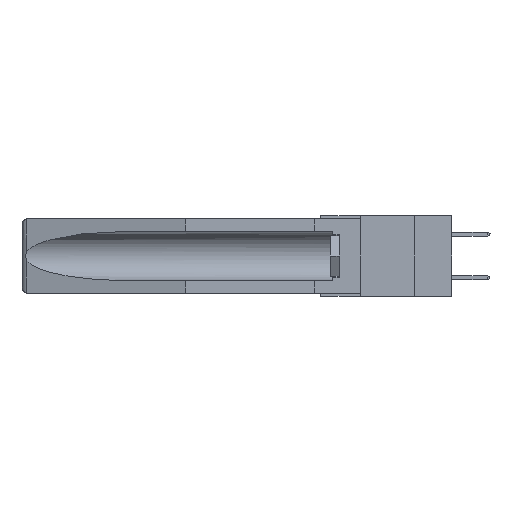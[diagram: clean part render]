
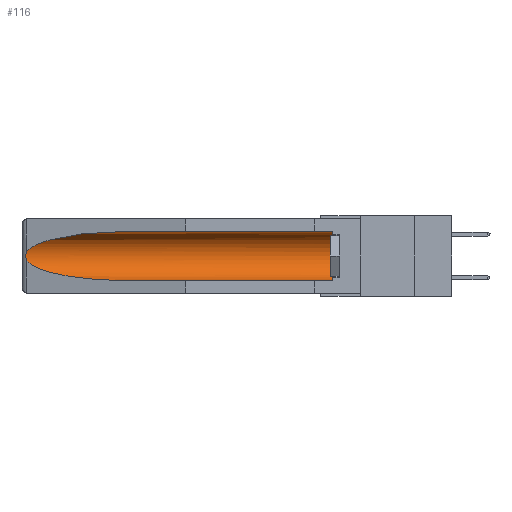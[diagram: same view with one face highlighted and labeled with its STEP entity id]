
A CAD part, left-side view. The second image highlights one B-rep face of the part: STEP entity #116.
In plain terms, the highlighted cylindrical face has radius 2.857 mm (diameter 5.715 mm), a partial arc.
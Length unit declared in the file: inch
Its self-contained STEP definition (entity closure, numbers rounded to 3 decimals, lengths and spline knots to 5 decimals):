
#116 = ADVANCED_FACE ( 'NONE', ( #16379 ), #17398, .F. ) ;
#505 = LINE ( 'NONE', #21112, #28038 ) ;
#758 = CARTESIAN_POINT ( 'NONE',  ( 0.155, 1.07973, -0.059 ) ) ;
#1160 = ORIENTED_EDGE ( 'NONE', *, *, #16626, .T. ) ;
#1648 = ORIENTED_EDGE ( 'NONE', *, *, #6688, .T. ) ;
#2032 = CARTESIAN_POINT ( 'NONE',  ( 0.26597, 1.52961, -0.15275 ) ) ;
#3458 = VECTOR ( 'NONE', #4696, 39.37008 ) ;
#4696 = DIRECTION ( 'NONE',  ( 0., 1., 0. ) ) ;
#4739 = CARTESIAN_POINT ( 'NONE',  ( 0.26537, 1.52718, -0.14972 ) ) ;
#4841 = CARTESIAN_POINT ( 'NONE',  ( 0.25451, 1.48313, -0.09465 ) ) ;
#4884 = DIRECTION ( 'NONE',  ( 0., 1., 0. ) ) ;
#5004 = CARTESIAN_POINT ( 'NONE',  ( 0.155, 0.126, -0.284 ) ) ;
#5081 = CARTESIAN_POINT ( 'NONE',  ( 0.26537, 1.52718, -0.19328 ) ) ;
#5505 = B_SPLINE_CURVE_WITH_KNOTS ( 'NONE', 3,
 ( #17147, #2032, #23636, #8386, #25745, #25563, #6096, #12748, #19293, #25662 ),
 .UNSPECIFIED., .F., .F.,
 ( 4, 2, 2, 2, 4 ),
 ( 0., 0.00029, 0.00058, 0.00087, 0.00117 ),
 .UNSPECIFIED. ) ;
#6096 = CARTESIAN_POINT ( 'NONE',  ( 0.2673, 1.53269, -0.17917 ) ) ;
#6135 = DIRECTION ( 'NONE',  ( 0., 1., 0. ) ) ;
#6383 =( BOUNDED_CURVE ( )  B_SPLINE_CURVE ( 3, ( #5081, #18288, #22518, #26839 ),
 .UNSPECIFIED., .F., .F. ) 
 B_SPLINE_CURVE_WITH_KNOTS ( ( 4, 4 ),
 ( 0.1948, 1.5708 ),
 .UNSPECIFIED. ) 
 CURVE ( )  GEOMETRIC_REPRESENTATION_ITEM ( )  RATIONAL_B_SPLINE_CURVE ( ( 1., 0.848, 0.848, 1. ) ) 
 REPRESENTATION_ITEM ( '' )  );
#6688 = EDGE_CURVE ( 'NONE', #25162, #22216, #5505, .T. ) ;
#8386 = CARTESIAN_POINT ( 'NONE',  ( 0.2673, 1.5327, -0.16383 ) ) ;
#8889 = CARTESIAN_POINT ( 'NONE',  ( 0.155, 1.07973, -0.284 ) ) ;
#9176 = CARTESIAN_POINT ( 'NONE',  ( 0.155, -0.30754, -0.284 ) ) ;
#9780 = EDGE_CURVE ( 'NONE', #26423, #22267, #20772, .T. ) ;
#10099 = CARTESIAN_POINT ( 'NONE',  ( 0.155, 0.126, -0.1715 ) ) ;
#11202 = EDGE_LOOP ( 'NONE', ( #24046, #1648, #1160, #26458, #12080, #26359 ) ) ;
#11216 = EDGE_CURVE ( 'NONE', #26423, #13217, #16270, .T. ) ;
#11830 = AXIS2_PLACEMENT_3D ( 'NONE', #10099, #12083, #25280 ) ;
#12080 = ORIENTED_EDGE ( 'NONE', *, *, #11216, .T. ) ;
#12083 = DIRECTION ( 'NONE',  ( 0., -1., 0. ) ) ;
#12748 = CARTESIAN_POINT ( 'NONE',  ( 0.26655, 1.53094, -0.18657 ) ) ;
#13217 = VERTEX_POINT ( 'NONE', #19183 ) ;
#13971 = EDGE_CURVE ( 'NONE', #13217, #21635, #505, .T. ) ;
#14360 = AXIS2_PLACEMENT_3D ( 'NONE', #19964, #4884, #22046 ) ;
#16270 = CIRCLE ( 'NONE', #11830, 0.1125 ) ;
#16379 = FACE_OUTER_BOUND ( 'NONE', #11202, .T. ) ;
#16626 = EDGE_CURVE ( 'NONE', #22216, #22267, #6383, .T. ) ;
#17147 = CARTESIAN_POINT ( 'NONE',  ( 0.26537, 1.52718, -0.14972 ) ) ;
#17398 = CYLINDRICAL_SURFACE ( 'NONE', #14360, 0.1125 ) ;
#17534 = CARTESIAN_POINT ( 'NONE',  ( 0.26537, 1.52718, -0.14972 ) ) ;
#18288 = CARTESIAN_POINT ( 'NONE',  ( 0.25451, 1.48313, -0.24835 ) ) ;
#18678 = CARTESIAN_POINT ( 'NONE',  ( 0.26537, 1.52718, -0.19328 ) ) ;
#19183 = CARTESIAN_POINT ( 'NONE',  ( 0.155, 0.126, -0.059 ) ) ;
#19293 = CARTESIAN_POINT ( 'NONE',  ( 0.26597, 1.5296, -0.19026 ) ) ;
#19428 =( BOUNDED_CURVE ( )  B_SPLINE_CURVE ( 3, ( #758, #20199, #4841, #4739 ),
 .UNSPECIFIED., .F., .F. ) 
 B_SPLINE_CURVE_WITH_KNOTS ( ( 4, 4 ),
 ( 4.71239, 6.08839 ),
 .UNSPECIFIED. ) 
 CURVE ( )  GEOMETRIC_REPRESENTATION_ITEM ( )  RATIONAL_B_SPLINE_CURVE ( ( 1., 0.848, 0.848, 1. ) ) 
 REPRESENTATION_ITEM ( '' )  );
#19964 = CARTESIAN_POINT ( 'NONE',  ( 0.155, -0.30754, -0.1715 ) ) ;
#20199 = CARTESIAN_POINT ( 'NONE',  ( 0.21114, 1.30732, -0.059 ) ) ;
#20772 = LINE ( 'NONE', #9176, #3458 ) ;
#21112 = CARTESIAN_POINT ( 'NONE',  ( 0.155, -0.30754, -0.059 ) ) ;
#21635 = VERTEX_POINT ( 'NONE', #23107 ) ;
#22046 = DIRECTION ( 'NONE',  ( 0., 0., 1. ) ) ;
#22216 = VERTEX_POINT ( 'NONE', #18678 ) ;
#22267 = VERTEX_POINT ( 'NONE', #8889 ) ;
#22518 = CARTESIAN_POINT ( 'NONE',  ( 0.21114, 1.30732, -0.284 ) ) ;
#23107 = CARTESIAN_POINT ( 'NONE',  ( 0.155, 1.07973, -0.059 ) ) ;
#23636 = CARTESIAN_POINT ( 'NONE',  ( 0.26654, 1.53092, -0.15636 ) ) ;
#24046 = ORIENTED_EDGE ( 'NONE', *, *, #25977, .T. ) ;
#25162 = VERTEX_POINT ( 'NONE', #17534 ) ;
#25280 = DIRECTION ( 'NONE',  ( 0., 0., 1. ) ) ;
#25563 = CARTESIAN_POINT ( 'NONE',  ( 0.2675, 1.53308, -0.17534 ) ) ;
#25662 = CARTESIAN_POINT ( 'NONE',  ( 0.26537, 1.52718, -0.19328 ) ) ;
#25745 = CARTESIAN_POINT ( 'NONE',  ( 0.2675, 1.53308, -0.16763 ) ) ;
#25977 = EDGE_CURVE ( 'NONE', #21635, #25162, #19428, .T. ) ;
#26359 = ORIENTED_EDGE ( 'NONE', *, *, #13971, .T. ) ;
#26423 = VERTEX_POINT ( 'NONE', #5004 ) ;
#26458 = ORIENTED_EDGE ( 'NONE', *, *, #9780, .F. ) ;
#26839 = CARTESIAN_POINT ( 'NONE',  ( 0.155, 1.07973, -0.284 ) ) ;
#28038 = VECTOR ( 'NONE', #6135, 39.37008 ) ;
